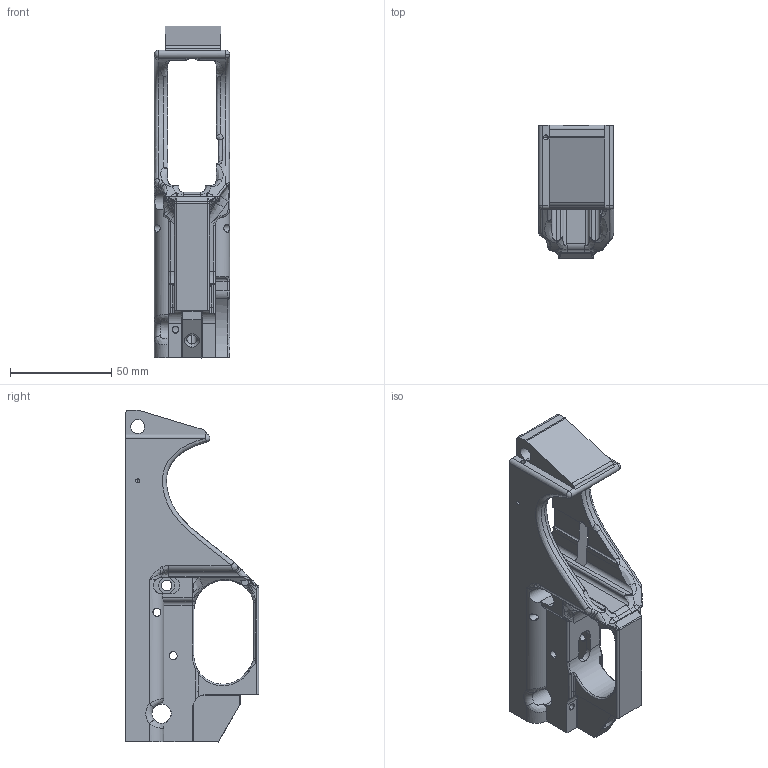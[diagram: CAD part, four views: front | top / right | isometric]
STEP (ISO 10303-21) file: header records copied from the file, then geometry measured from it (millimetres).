
FILE_DESCRIPTION (( 'STEP AP214' ), '1' );
FILE_NAME ('Hermes_v1.4_Front.STEP', '2015-05-21T07:11:49', ( 'WarFairy' ), ( '' ), 'SwSTEP 2.0', 'SolidWorks 2015', '' );
FILE_SCHEMA (( 'AUTOMOTIVE_DESIGN' ));
Length unit declared in the file: inch
Products named in the file (1): Hermes_v1.4_Front
Bounding box: 37.13 x 65.79 x 163.69 mm (x, y, z)
Volume: 101444.8 mm3; surface area: 40310.5 mm2
Topology: 1 solids, 3 shells, 395 faces, 1069 edges, 649 vertices
Faces by surface type: cylinder 145, bspline 121, plane 91, torus 24, sphere 8, cone 6
Entity records: 24522 total; most frequent: CARTESIAN_POINT 15617, ORIENTED_EDGE 2092, DIRECTION 1550, EDGE_CURVE 1046, VERTEX_POINT 649, AXIS2_PLACEMENT_3D 584, EDGE_LOOP 419, FACE_OUTER_BOUND 395
